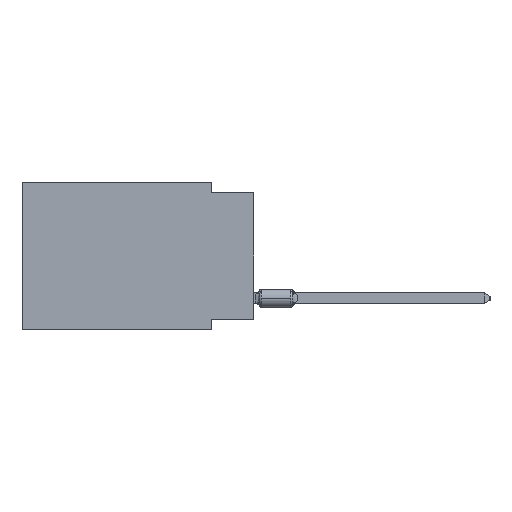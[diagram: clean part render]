
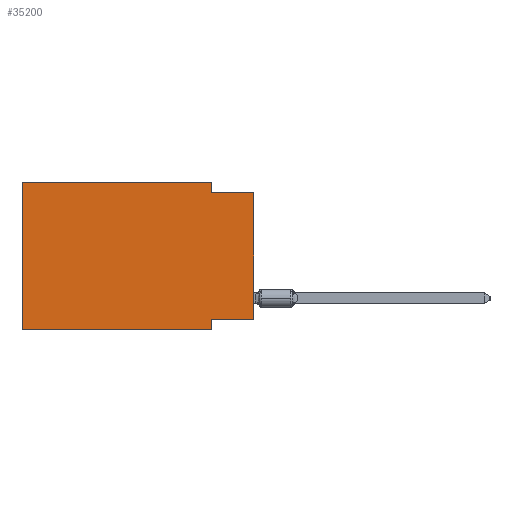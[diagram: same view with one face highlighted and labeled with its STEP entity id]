
A CAD part, left-side view. The second image highlights one B-rep face of the part: STEP entity #35200.
In plain terms, the highlighted planar face has unit normal (-1, 0, 0).
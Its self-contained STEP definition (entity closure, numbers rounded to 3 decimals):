
#4020 = LINE ( 'NONE', #33485, #46919 ) ;
#4735 = VERTEX_POINT ( 'NONE', #14987 ) ;
#5371 = VECTOR ( 'NONE', #58366, 1000. ) ;
#6141 = LINE ( 'NONE', #50664, #28674 ) ;
#6881 = EDGE_CURVE ( 'NONE', #36695, #26770, #55354, .T. ) ;
#7235 = EDGE_CURVE ( 'NONE', #37952, #45354, #13719, .T. ) ;
#7938 = LINE ( 'NONE', #17424, #5371 ) ;
#8787 = VECTOR ( 'NONE', #11589, 1000. ) ;
#11284 = VERTEX_POINT ( 'NONE', #52323 ) ;
#11589 = DIRECTION ( 'NONE',  ( 0., 0., 1. ) ) ;
#13056 = PLANE ( 'NONE',  #29818 ) ;
#13706 = DIRECTION ( 'NONE',  ( 0., 0., -1. ) ) ;
#13719 = LINE ( 'NONE', #54625, #57717 ) ;
#14765 = CARTESIAN_POINT ( 'NONE',  ( 0., 0., -8.255 ) ) ;
#14987 = CARTESIAN_POINT ( 'NONE',  ( 0., 0., -0.635 ) ) ;
#16025 = ORIENTED_EDGE ( 'NONE', *, *, #36547, .F. ) ;
#16047 = ORIENTED_EDGE ( 'NONE', *, *, #51770, .T. ) ;
#16189 = VECTOR ( 'NONE', #42313, 1000. ) ;
#16258 = DIRECTION ( 'NONE',  ( 0., 0., -1. ) ) ;
#16358 = DIRECTION ( 'NONE',  ( 0., -1., 0. ) ) ;
#17424 = CARTESIAN_POINT ( 'NONE',  ( 0., 0., -8.255 ) ) ;
#19481 = ORIENTED_EDGE ( 'NONE', *, *, #6881, .T. ) ;
#23318 = ORIENTED_EDGE ( 'NONE', *, *, #28244, .F. ) ;
#26770 = VERTEX_POINT ( 'NONE', #46152 ) ;
#27099 = CARTESIAN_POINT ( 'NONE',  ( 0., 13.97, -8.89 ) ) ;
#27229 = CARTESIAN_POINT ( 'NONE',  ( 0., 13.97, 0. ) ) ;
#28244 = EDGE_CURVE ( 'NONE', #29616, #11284, #7938, .T. ) ;
#28674 = VECTOR ( 'NONE', #16258, 1000. ) ;
#29072 = DIRECTION ( 'NONE',  ( 1., 0., 0. ) ) ;
#29299 = ORIENTED_EDGE ( 'NONE', *, *, #34557, .F. ) ;
#29616 = VERTEX_POINT ( 'NONE', #14765 ) ;
#29711 = DIRECTION ( 'NONE',  ( 0., -1., 0. ) ) ;
#29818 = AXIS2_PLACEMENT_3D ( 'NONE', #43854, #29072, #13706 ) ;
#31029 = VERTEX_POINT ( 'NONE', #41553 ) ;
#31755 = CARTESIAN_POINT ( 'NONE',  ( 0., 13.97, -8.89 ) ) ;
#32458 = LINE ( 'NONE', #27229, #16189 ) ;
#33071 = EDGE_CURVE ( 'NONE', #36695, #31029, #36477, .T. ) ;
#33485 = CARTESIAN_POINT ( 'NONE',  ( 0., 0., 0. ) ) ;
#33677 = EDGE_CURVE ( 'NONE', #11284, #26770, #6141, .T. ) ;
#34557 = EDGE_CURVE ( 'NONE', #31029, #37952, #32458, .T. ) ;
#34761 = DIRECTION ( 'NONE',  ( 0., 0., 1. ) ) ;
#35200 = ADVANCED_FACE ( 'NONE', ( #58587 ), #13056, .F. ) ;
#36477 = LINE ( 'NONE', #56452, #8787 ) ;
#36547 = EDGE_CURVE ( 'NONE', #45354, #4735, #49710, .T. ) ;
#36695 = VERTEX_POINT ( 'NONE', #27099 ) ;
#37355 = VECTOR ( 'NONE', #29711, 1000. ) ;
#37952 = VERTEX_POINT ( 'NONE', #50775 ) ;
#39580 = DIRECTION ( 'NONE',  ( 0., 0., -1. ) ) ;
#41133 = EDGE_LOOP ( 'NONE', ( #16047, #16025, #45848, #29299, #45762, #19481, #46405, #23318 ) ) ;
#41553 = CARTESIAN_POINT ( 'NONE',  ( 0., 13.97, 0. ) ) ;
#42313 = DIRECTION ( 'NONE',  ( 0., -1., 0. ) ) ;
#43854 = CARTESIAN_POINT ( 'NONE',  ( 0., 13.97, 0. ) ) ;
#45140 = CARTESIAN_POINT ( 'NONE',  ( 0., 0., -0.635 ) ) ;
#45354 = VERTEX_POINT ( 'NONE', #48291 ) ;
#45762 = ORIENTED_EDGE ( 'NONE', *, *, #33071, .F. ) ;
#45848 = ORIENTED_EDGE ( 'NONE', *, *, #7235, .F. ) ;
#46152 = CARTESIAN_POINT ( 'NONE',  ( 0., 2.54, -8.89 ) ) ;
#46405 = ORIENTED_EDGE ( 'NONE', *, *, #33677, .F. ) ;
#46919 = VECTOR ( 'NONE', #34761, 1000. ) ;
#48291 = CARTESIAN_POINT ( 'NONE',  ( 0., 2.54, -0.635 ) ) ;
#49710 = LINE ( 'NONE', #45140, #37355 ) ;
#50664 = CARTESIAN_POINT ( 'NONE',  ( 0., 2.54, -8.89 ) ) ;
#50775 = CARTESIAN_POINT ( 'NONE',  ( 0., 2.54, 0. ) ) ;
#51770 = EDGE_CURVE ( 'NONE', #29616, #4735, #4020, .T. ) ;
#52323 = CARTESIAN_POINT ( 'NONE',  ( 0., 2.54, -8.255 ) ) ;
#54625 = CARTESIAN_POINT ( 'NONE',  ( 0., 2.54, 0. ) ) ;
#55354 = LINE ( 'NONE', #31755, #62968 ) ;
#56452 = CARTESIAN_POINT ( 'NONE',  ( 0., 13.97, 0. ) ) ;
#57717 = VECTOR ( 'NONE', #39580, 1000. ) ;
#58366 = DIRECTION ( 'NONE',  ( 0., 1., 0. ) ) ;
#58587 = FACE_OUTER_BOUND ( 'NONE', #41133, .T. ) ;
#62968 = VECTOR ( 'NONE', #16358, 1000. ) ;
